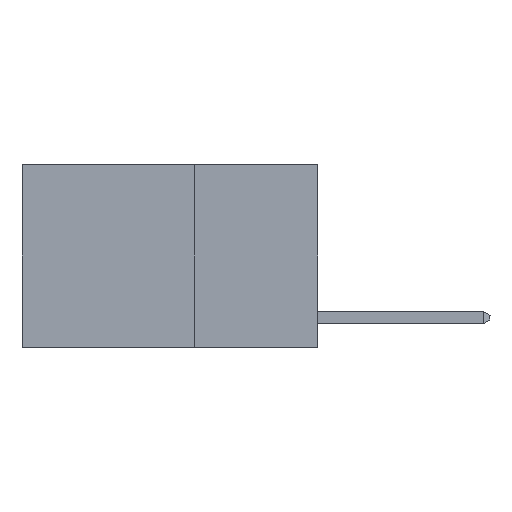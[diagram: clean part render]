
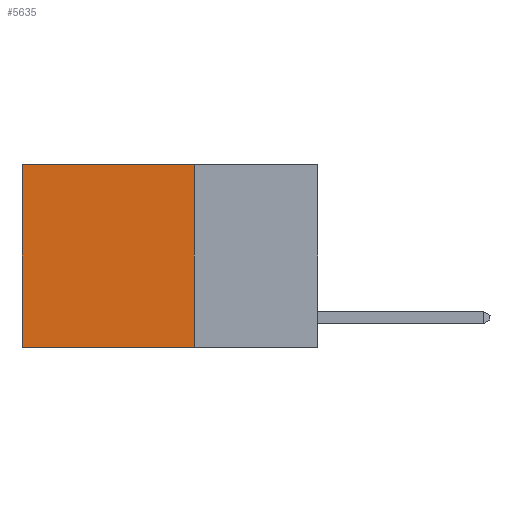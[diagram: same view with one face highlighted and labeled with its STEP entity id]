
A CAD part, left-side view. The second image highlights one B-rep face of the part: STEP entity #5635.
In plain terms, the highlighted planar face has unit normal (-1, 0, 0).
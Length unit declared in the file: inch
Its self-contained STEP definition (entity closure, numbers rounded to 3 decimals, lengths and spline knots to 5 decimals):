
#53 = VERTEX_POINT ( 'NONE', #4747 ) ;
#253 = ORIENTED_EDGE ( 'NONE', *, *, #2342, .F. ) ;
#558 = CARTESIAN_POINT ( 'NONE',  ( 0.2625, 0.25, -0.37 ) ) ;
#1009 = DIRECTION ( 'NONE',  ( 0., 0., -1. ) ) ;
#1060 = AXIS2_PLACEMENT_3D ( 'NONE', #11866, #7163, #8167 ) ;
#1223 = EDGE_LOOP ( 'NONE', ( #9044, #253, #3385, #2071 ) ) ;
#1545 = FACE_OUTER_BOUND ( 'NONE', #1223, .T. ) ;
#1986 = CARTESIAN_POINT ( 'NONE',  ( 0.2625, 0.25, 0. ) ) ;
#2071 = ORIENTED_EDGE ( 'NONE', *, *, #10051, .T. ) ;
#2342 = EDGE_CURVE ( 'NONE', #3666, #53, #3953, .T. ) ;
#2743 = VECTOR ( 'NONE', #9984, 39.37008 ) ;
#3023 = CARTESIAN_POINT ( 'NONE',  ( 0.2625, 0.25, 0. ) ) ;
#3113 = EDGE_CURVE ( 'NONE', #8409, #3666, #9102, .T. ) ;
#3385 = ORIENTED_EDGE ( 'NONE', *, *, #3113, .F. ) ;
#3666 = VERTEX_POINT ( 'NONE', #10975 ) ;
#3953 = LINE ( 'NONE', #558, #2743 ) ;
#4747 = CARTESIAN_POINT ( 'NONE',  ( 0.2625, 0.6, -0.37 ) ) ;
#5635 = ADVANCED_FACE ( 'NONE', ( #1545 ), #6237, .F. ) ;
#6237 = PLANE ( 'NONE',  #1060 ) ;
#7163 = DIRECTION ( 'NONE',  ( 1., 0., 0. ) ) ;
#7520 = CARTESIAN_POINT ( 'NONE',  ( 0.2625, 0.6, 0. ) ) ;
#7587 = CARTESIAN_POINT ( 'NONE',  ( 0.2625, 0.25, 0. ) ) ;
#7845 = EDGE_CURVE ( 'NONE', #9877, #53, #11083, .T. ) ;
#8167 = DIRECTION ( 'NONE',  ( 0., 0., -1. ) ) ;
#8409 = VERTEX_POINT ( 'NONE', #3023 ) ;
#8634 = DIRECTION ( 'NONE',  ( 0., 1., 0. ) ) ;
#9044 = ORIENTED_EDGE ( 'NONE', *, *, #7845, .T. ) ;
#9054 = CARTESIAN_POINT ( 'NONE',  ( 0.2625, 0.6, 0. ) ) ;
#9102 = LINE ( 'NONE', #1986, #11336 ) ;
#9877 = VERTEX_POINT ( 'NONE', #9054 ) ;
#9984 = DIRECTION ( 'NONE',  ( 0., 1., 0. ) ) ;
#10051 = EDGE_CURVE ( 'NONE', #8409, #9877, #11484, .T. ) ;
#10248 = DIRECTION ( 'NONE',  ( 0., 0., -1. ) ) ;
#10886 = VECTOR ( 'NONE', #8634, 39.37008 ) ;
#10975 = CARTESIAN_POINT ( 'NONE',  ( 0.2625, 0.25, -0.37 ) ) ;
#11083 = LINE ( 'NONE', #7520, #11390 ) ;
#11336 = VECTOR ( 'NONE', #1009, 39.37008 ) ;
#11390 = VECTOR ( 'NONE', #10248, 39.37008 ) ;
#11484 = LINE ( 'NONE', #7587, #10886 ) ;
#11866 = CARTESIAN_POINT ( 'NONE',  ( 0.2625, 0.25, 0. ) ) ;
